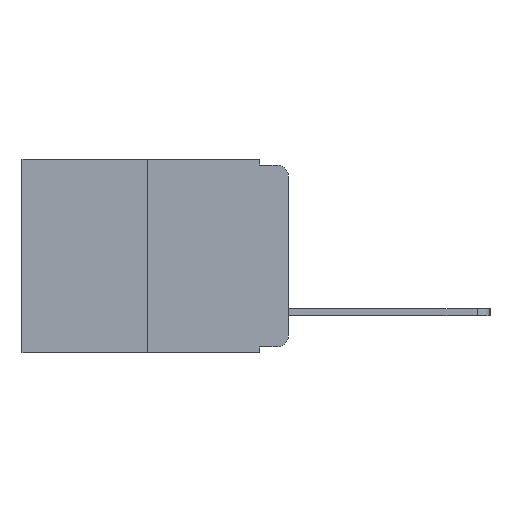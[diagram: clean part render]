
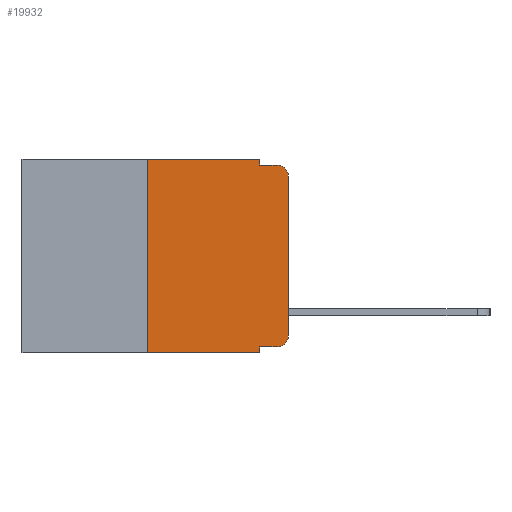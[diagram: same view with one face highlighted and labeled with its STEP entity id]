
A CAD part, left-side view. The second image highlights one B-rep face of the part: STEP entity #19932.
In plain terms, the highlighted planar face has unit normal (-1, 0, 0).
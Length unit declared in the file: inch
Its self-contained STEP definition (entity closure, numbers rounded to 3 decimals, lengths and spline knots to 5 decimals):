
#361 = VERTEX_POINT ( 'NONE', #7518 ) ;
#384 = CARTESIAN_POINT ( 'NONE',  ( 0., 0.051, -0.333 ) ) ;
#435 = DIRECTION ( 'NONE',  ( 0., -1., 0. ) ) ;
#509 = VERTEX_POINT ( 'NONE', #6939 ) ;
#943 = ORIENTED_EDGE ( 'NONE', *, *, #7952, .T. ) ;
#965 = VERTEX_POINT ( 'NONE', #1726 ) ;
#976 = EDGE_CURVE ( 'NONE', #11289, #12164, #17381, .T. ) ;
#1405 = VECTOR ( 'NONE', #10007, 39.37008 ) ;
#1624 = DIRECTION ( 'NONE',  ( 0., 0., -1. ) ) ;
#1726 = CARTESIAN_POINT ( 'NONE',  ( 0., 0.051, -0.01 ) ) ;
#2604 = VECTOR ( 'NONE', #435, 39.37008 ) ;
#2653 = VECTOR ( 'NONE', #18848, 39.37008 ) ;
#3072 = CARTESIAN_POINT ( 'NONE',  ( 0., 0.051, 0. ) ) ;
#3277 = PLANE ( 'NONE',  #19605 ) ;
#3297 = CARTESIAN_POINT ( 'NONE',  ( 0., 0.473, 0. ) ) ;
#3696 = CARTESIAN_POINT ( 'NONE',  ( 0., 0.25, -0.343 ) ) ;
#4148 = AXIS2_PLACEMENT_3D ( 'NONE', #5900, #5825, #5749 ) ;
#4916 = LINE ( 'NONE', #3072, #12437 ) ;
#5387 = EDGE_CURVE ( 'NONE', #17195, #11289, #15284, .T. ) ;
#5749 = DIRECTION ( 'NONE',  ( 0., 0., -1. ) ) ;
#5767 = EDGE_CURVE ( 'NONE', #361, #16036, #14063, .T. ) ;
#5825 = DIRECTION ( 'NONE',  ( -1., 0., 0. ) ) ;
#5900 = CARTESIAN_POINT ( 'NONE',  ( 0., 0.02, -0.313 ) ) ;
#6025 = VECTOR ( 'NONE', #14912, 39.37008 ) ;
#6110 = CARTESIAN_POINT ( 'NONE',  ( 0., 0.25, 0. ) ) ;
#6404 = DIRECTION ( 'NONE',  ( 1., 0., 0. ) ) ;
#6939 = CARTESIAN_POINT ( 'NONE',  ( 0., 0.051, -0.333 ) ) ;
#7118 = VERTEX_POINT ( 'NONE', #15915 ) ;
#7141 = EDGE_CURVE ( 'NONE', #12164, #965, #9707, .T. ) ;
#7149 = CARTESIAN_POINT ( 'NONE',  ( 0., 0., 0. ) ) ;
#7237 = VECTOR ( 'NONE', #15348, 39.37008 ) ;
#7518 = CARTESIAN_POINT ( 'NONE',  ( 0., 0., -0.313 ) ) ;
#7952 = EDGE_CURVE ( 'NONE', #16036, #7118, #12964, .T. ) ;
#8364 = EDGE_CURVE ( 'NONE', #14666, #361, #10752, .T. ) ;
#8457 = EDGE_CURVE ( 'NONE', #509, #19007, #4916, .T. ) ;
#8602 = ORIENTED_EDGE ( 'NONE', *, *, #15020, .T. ) ;
#9707 = LINE ( 'NONE', #16757, #13283 ) ;
#10007 = DIRECTION ( 'NONE',  ( 0., -1., 0. ) ) ;
#10129 = LINE ( 'NONE', #17704, #1405 ) ;
#10178 = ORIENTED_EDGE ( 'NONE', *, *, #7141, .F. ) ;
#10225 = FACE_OUTER_BOUND ( 'NONE', #14970, .T. ) ;
#10587 = EDGE_CURVE ( 'NONE', #509, #14666, #14880, .T. ) ;
#10673 = LINE ( 'NONE', #11248, #2604 ) ;
#10752 = CIRCLE ( 'NONE', #4148, 0.02 ) ;
#11248 = CARTESIAN_POINT ( 'NONE',  ( 0., 0.051, -0.01 ) ) ;
#11289 = VERTEX_POINT ( 'NONE', #16299 ) ;
#12164 = VERTEX_POINT ( 'NONE', #15171 ) ;
#12437 = VECTOR ( 'NONE', #1624, 39.37008 ) ;
#12964 = CIRCLE ( 'NONE', #15748, 0.02 ) ;
#12990 = CARTESIAN_POINT ( 'NONE',  ( 0., 0., -0.03 ) ) ;
#13159 = CARTESIAN_POINT ( 'NONE',  ( 0., 0.02, -0.333 ) ) ;
#13255 = VECTOR ( 'NONE', #13835, 39.37008 ) ;
#13283 = VECTOR ( 'NONE', #17321, 39.37008 ) ;
#13303 = ORIENTED_EDGE ( 'NONE', *, *, #15996, .F. ) ;
#13835 = DIRECTION ( 'NONE',  ( 0., -1., 0. ) ) ;
#14063 = LINE ( 'NONE', #7149, #6025 ) ;
#14666 = VERTEX_POINT ( 'NONE', #13159 ) ;
#14880 = LINE ( 'NONE', #384, #2653 ) ;
#14912 = DIRECTION ( 'NONE',  ( 0., 0., 1. ) ) ;
#14970 = EDGE_LOOP ( 'NONE', ( #19943, #943, #13303, #10178, #18800, #15729, #8602, #17198, #18152, #19048 ) ) ;
#15020 = EDGE_CURVE ( 'NONE', #17195, #19007, #10129, .T. ) ;
#15171 = CARTESIAN_POINT ( 'NONE',  ( 0., 0.051, 0. ) ) ;
#15284 = LINE ( 'NONE', #6110, #7237 ) ;
#15348 = DIRECTION ( 'NONE',  ( 0., 0., 1. ) ) ;
#15484 = CARTESIAN_POINT ( 'NONE',  ( 0., 0.473, 0. ) ) ;
#15729 = ORIENTED_EDGE ( 'NONE', *, *, #5387, .F. ) ;
#15748 = AXIS2_PLACEMENT_3D ( 'NONE', #18293, #18175, #17230 ) ;
#15915 = CARTESIAN_POINT ( 'NONE',  ( 0., 0.02, -0.01 ) ) ;
#15996 = EDGE_CURVE ( 'NONE', #965, #7118, #10673, .T. ) ;
#16036 = VERTEX_POINT ( 'NONE', #12990 ) ;
#16299 = CARTESIAN_POINT ( 'NONE',  ( 0., 0.25, 0. ) ) ;
#16757 = CARTESIAN_POINT ( 'NONE',  ( 0., 0.051, 0. ) ) ;
#17060 = DIRECTION ( 'NONE',  ( 0., 0., -1. ) ) ;
#17195 = VERTEX_POINT ( 'NONE', #3696 ) ;
#17198 = ORIENTED_EDGE ( 'NONE', *, *, #8457, .F. ) ;
#17230 = DIRECTION ( 'NONE',  ( 0., 0., -1. ) ) ;
#17321 = DIRECTION ( 'NONE',  ( 0., 0., -1. ) ) ;
#17381 = LINE ( 'NONE', #3297, #13255 ) ;
#17503 = CARTESIAN_POINT ( 'NONE',  ( 0., 0.051, -0.343 ) ) ;
#17704 = CARTESIAN_POINT ( 'NONE',  ( 0., 0.473, -0.343 ) ) ;
#18152 = ORIENTED_EDGE ( 'NONE', *, *, #10587, .T. ) ;
#18175 = DIRECTION ( 'NONE',  ( -1., 0., 0. ) ) ;
#18293 = CARTESIAN_POINT ( 'NONE',  ( 0., 0.02, -0.03 ) ) ;
#18800 = ORIENTED_EDGE ( 'NONE', *, *, #976, .F. ) ;
#18848 = DIRECTION ( 'NONE',  ( 0., -1., 0. ) ) ;
#19007 = VERTEX_POINT ( 'NONE', #17503 ) ;
#19048 = ORIENTED_EDGE ( 'NONE', *, *, #8364, .T. ) ;
#19605 = AXIS2_PLACEMENT_3D ( 'NONE', #15484, #6404, #17060 ) ;
#19932 = ADVANCED_FACE ( 'NONE', ( #10225 ), #3277, .F. ) ;
#19943 = ORIENTED_EDGE ( 'NONE', *, *, #5767, .T. ) ;
